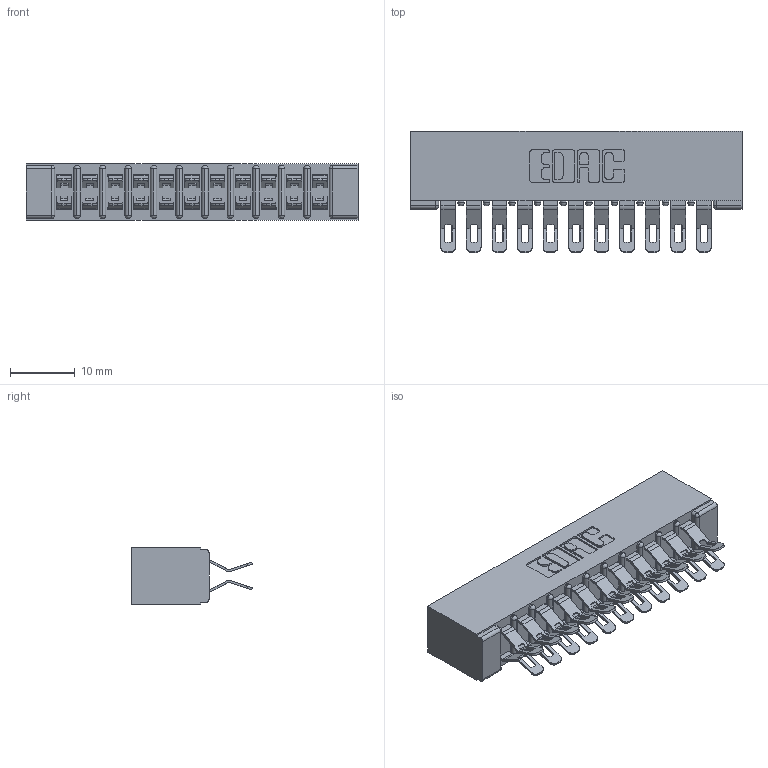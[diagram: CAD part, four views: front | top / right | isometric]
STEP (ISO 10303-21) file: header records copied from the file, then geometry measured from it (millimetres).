
FILE_DESCRIPTION (( 'STEP AP203' ), '1' );
FILE_NAME ('357-022-455-201.STEP', '2020-10-02T23:37:47', ( '' ), ( '' ), 'SwSTEP 2.0', 'SolidWorks 2020', '' );
FILE_SCHEMA (( 'CONFIG_CONTROL_DESIGN' ));
Length unit declared in the file: inch
Products named in the file (3): 307 Part_No Mounting Lugs; 307-290-001_555; 357-022-455-201
Assembly tree (23 placements, depth 2):
  357-022-455-201
    307 Part_No Mounting Lugs
    307-290-001_555  x22
Bounding box: 51.46 x 18.75 x 8.71 mm (x, y, z)
Volume: 3666 mm3; surface area: 6734 mm2
Topology: 23 solids, 23 shells, 1464 faces, 4281 edges, 2790 vertices
Faces by surface type: plane 814, cylinder 626, sphere 24
Entity records: 13863 total; most frequent: CARTESIAN_POINT 2279, ORIENTED_EDGE 2256, DIRECTION 2252, EDGE_CURVE 1128, LINE 842, VECTOR 842, VERTEX_POINT 732, AXIS2_PLACEMENT_3D 705
